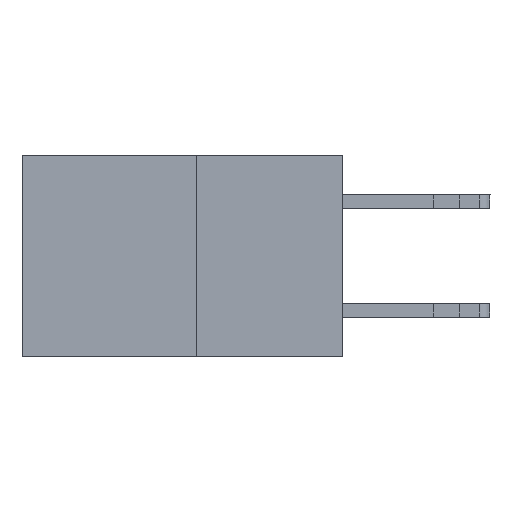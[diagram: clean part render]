
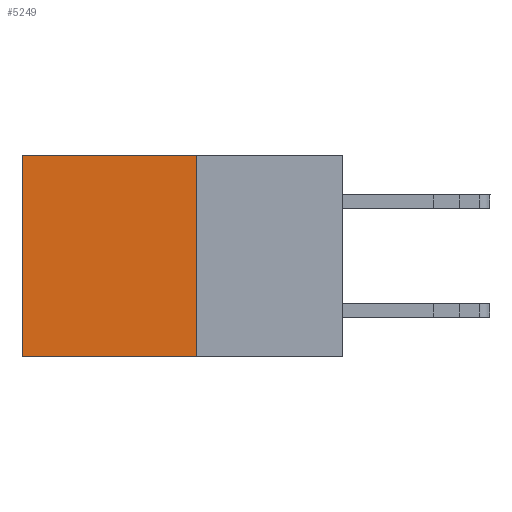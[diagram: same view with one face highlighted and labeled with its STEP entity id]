
A CAD part, left-side view. The second image highlights one B-rep face of the part: STEP entity #5249.
In plain terms, the highlighted planar face has unit normal (-1, 0, 0).
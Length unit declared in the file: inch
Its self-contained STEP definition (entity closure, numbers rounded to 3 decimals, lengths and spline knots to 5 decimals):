
#41 = VECTOR ( 'NONE', #3179, 39.37008 ) ;
#660 = DIRECTION ( 'NONE',  ( 0., 0., -1. ) ) ;
#736 = ORIENTED_EDGE ( 'NONE', *, *, #8238, .T. ) ;
#1786 = CARTESIAN_POINT ( 'NONE',  ( 0.277, 0.59, -0.37 ) ) ;
#2041 = CARTESIAN_POINT ( 'NONE',  ( 0.277, 0.59, -0.37 ) ) ;
#2177 = LINE ( 'NONE', #5092, #4500 ) ;
#2640 = EDGE_CURVE ( 'NONE', #4965, #12398, #7998, .T. ) ;
#3179 = DIRECTION ( 'NONE',  ( 0., 0., -1. ) ) ;
#3689 = ORIENTED_EDGE ( 'NONE', *, *, #9735, .T. ) ;
#3854 = CARTESIAN_POINT ( 'NONE',  ( 0.277, 0.27, -0.37 ) ) ;
#4215 = VECTOR ( 'NONE', #11943, 39.37008 ) ;
#4458 = AXIS2_PLACEMENT_3D ( 'NONE', #4615, #11658, #660 ) ;
#4500 = VECTOR ( 'NONE', #9103, 39.37008 ) ;
#4611 = CARTESIAN_POINT ( 'NONE',  ( 0.277, 0.27, -0.37 ) ) ;
#4615 = CARTESIAN_POINT ( 'NONE',  ( 0.277, 0.27, -0.37 ) ) ;
#4965 = VERTEX_POINT ( 'NONE', #11855 ) ;
#5092 = CARTESIAN_POINT ( 'NONE',  ( 0.277, 0.27, 0. ) ) ;
#5249 = ADVANCED_FACE ( 'NONE', ( #12748 ), #9554, .F. ) ;
#5635 = LINE ( 'NONE', #4611, #12244 ) ;
#5980 = VERTEX_POINT ( 'NONE', #12459 ) ;
#5997 = LINE ( 'NONE', #2041, #41 ) ;
#6727 = VERTEX_POINT ( 'NONE', #8969 ) ;
#7998 = LINE ( 'NONE', #3854, #4215 ) ;
#8238 = EDGE_CURVE ( 'NONE', #6727, #5980, #2177, .T. ) ;
#8251 = ORIENTED_EDGE ( 'NONE', *, *, #11376, .F. ) ;
#8969 = CARTESIAN_POINT ( 'NONE',  ( 0.277, 0.27, 0. ) ) ;
#9103 = DIRECTION ( 'NONE',  ( 0., 1., 0. ) ) ;
#9425 = EDGE_LOOP ( 'NONE', ( #3689, #12533, #8251, #736 ) ) ;
#9554 = PLANE ( 'NONE',  #4458 ) ;
#9735 = EDGE_CURVE ( 'NONE', #5980, #12398, #5997, .T. ) ;
#11376 = EDGE_CURVE ( 'NONE', #6727, #4965, #5635, .T. ) ;
#11658 = DIRECTION ( 'NONE',  ( 1., 0., 0. ) ) ;
#11855 = CARTESIAN_POINT ( 'NONE',  ( 0.277, 0.27, -0.37 ) ) ;
#11943 = DIRECTION ( 'NONE',  ( 0., 1., 0. ) ) ;
#12244 = VECTOR ( 'NONE', #12799, 39.37008 ) ;
#12398 = VERTEX_POINT ( 'NONE', #1786 ) ;
#12459 = CARTESIAN_POINT ( 'NONE',  ( 0.277, 0.59, 0. ) ) ;
#12533 = ORIENTED_EDGE ( 'NONE', *, *, #2640, .F. ) ;
#12748 = FACE_OUTER_BOUND ( 'NONE', #9425, .T. ) ;
#12799 = DIRECTION ( 'NONE',  ( 0., 0., -1. ) ) ;
